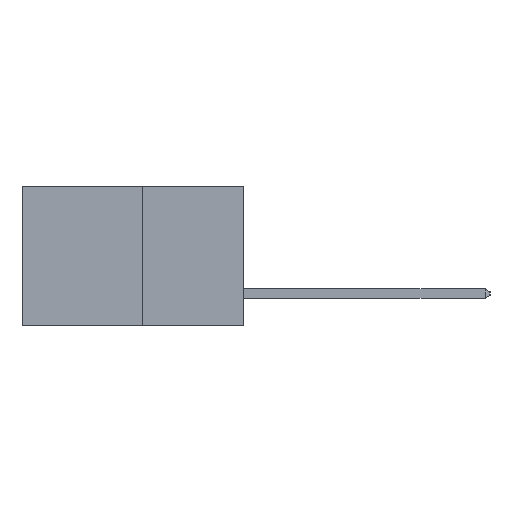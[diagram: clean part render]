
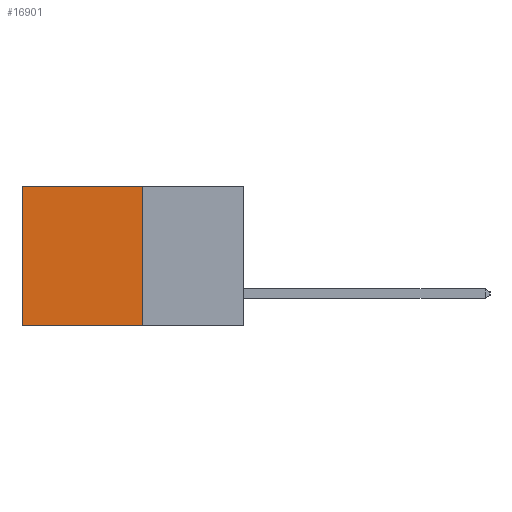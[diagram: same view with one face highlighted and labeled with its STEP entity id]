
A CAD part, left-side view. The second image highlights one B-rep face of the part: STEP entity #16901.
In plain terms, the highlighted planar face has unit normal (-1, 0, 0).
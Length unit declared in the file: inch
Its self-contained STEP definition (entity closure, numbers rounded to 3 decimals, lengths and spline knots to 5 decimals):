
#109 = EDGE_CURVE ( 'NONE', #10956, #10263, #14144, .T. ) ;
#407 = ORIENTED_EDGE ( 'NONE', *, *, #13583, .T. ) ;
#654 = DIRECTION ( 'NONE',  ( 0., 0., -1. ) ) ;
#686 = CARTESIAN_POINT ( 'NONE',  ( 0.277, 0.59, -0.37 ) ) ;
#1070 = VECTOR ( 'NONE', #654, 39.37008 ) ;
#1331 = VERTEX_POINT ( 'NONE', #10481 ) ;
#3162 = VECTOR ( 'NONE', #14850, 39.37008 ) ;
#4287 = DIRECTION ( 'NONE',  ( 1., 0., 0. ) ) ;
#4347 = VERTEX_POINT ( 'NONE', #14220 ) ;
#4481 = EDGE_CURVE ( 'NONE', #10956, #1331, #10598, .T. ) ;
#5470 = EDGE_LOOP ( 'NONE', ( #407, #11982, #13217, #14049 ) ) ;
#5542 = EDGE_CURVE ( 'NONE', #1331, #4347, #17225, .T. ) ;
#6531 = FACE_OUTER_BOUND ( 'NONE', #5470, .T. ) ;
#7074 = PLANE ( 'NONE',  #16801 ) ;
#7760 = CARTESIAN_POINT ( 'NONE',  ( 0.277, 0.27, 0. ) ) ;
#8554 = CARTESIAN_POINT ( 'NONE',  ( 0.277, 0.59, 0. ) ) ;
#8981 = LINE ( 'NONE', #686, #1070 ) ;
#10125 = VECTOR ( 'NONE', #11962, 39.37008 ) ;
#10263 = VERTEX_POINT ( 'NONE', #8554 ) ;
#10481 = CARTESIAN_POINT ( 'NONE',  ( 0.277, 0.27, -0.37 ) ) ;
#10598 = LINE ( 'NONE', #11306, #17729 ) ;
#10956 = VERTEX_POINT ( 'NONE', #17243 ) ;
#11306 = CARTESIAN_POINT ( 'NONE',  ( 0.277, 0.27, -0.37 ) ) ;
#11857 = CARTESIAN_POINT ( 'NONE',  ( 0.277, 0.27, -0.37 ) ) ;
#11881 = DIRECTION ( 'NONE',  ( 0., 0., -1. ) ) ;
#11962 = DIRECTION ( 'NONE',  ( 0., 1., 0. ) ) ;
#11982 = ORIENTED_EDGE ( 'NONE', *, *, #5542, .F. ) ;
#12553 = CARTESIAN_POINT ( 'NONE',  ( 0.277, 0.27, -0.37 ) ) ;
#13217 = ORIENTED_EDGE ( 'NONE', *, *, #4481, .F. ) ;
#13583 = EDGE_CURVE ( 'NONE', #10263, #4347, #8981, .T. ) ;
#13881 = DIRECTION ( 'NONE',  ( 0., 0., -1. ) ) ;
#14049 = ORIENTED_EDGE ( 'NONE', *, *, #109, .T. ) ;
#14144 = LINE ( 'NONE', #7760, #3162 ) ;
#14220 = CARTESIAN_POINT ( 'NONE',  ( 0.277, 0.59, -0.37 ) ) ;
#14850 = DIRECTION ( 'NONE',  ( 0., 1., 0. ) ) ;
#16801 = AXIS2_PLACEMENT_3D ( 'NONE', #12553, #4287, #13881 ) ;
#16901 = ADVANCED_FACE ( 'NONE', ( #6531 ), #7074, .F. ) ;
#17225 = LINE ( 'NONE', #11857, #10125 ) ;
#17243 = CARTESIAN_POINT ( 'NONE',  ( 0.277, 0.27, 0. ) ) ;
#17729 = VECTOR ( 'NONE', #11881, 39.37008 ) ;
